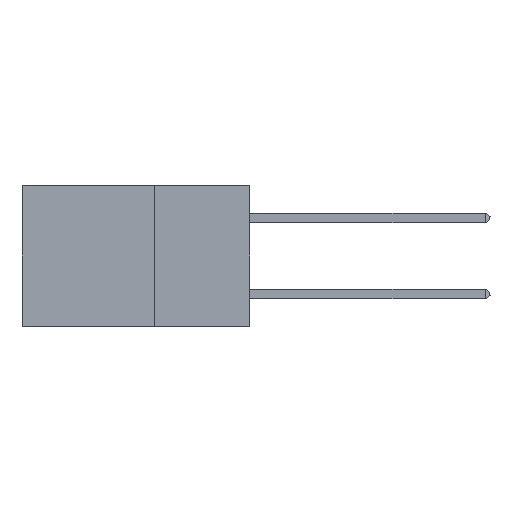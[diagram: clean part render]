
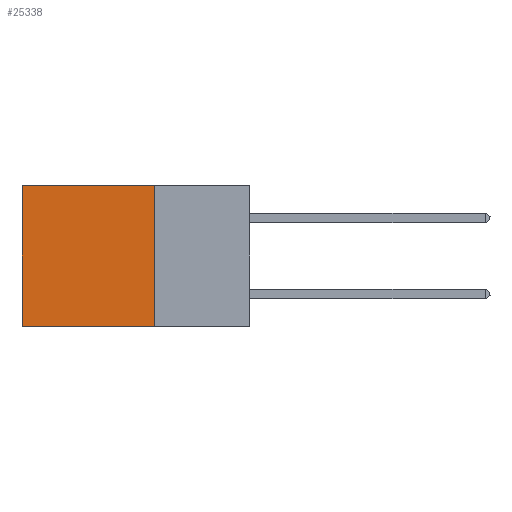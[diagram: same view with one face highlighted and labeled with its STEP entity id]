
A CAD part, left-side view. The second image highlights one B-rep face of the part: STEP entity #25338.
In plain terms, the highlighted planar face has unit normal (-1, 0, 0).
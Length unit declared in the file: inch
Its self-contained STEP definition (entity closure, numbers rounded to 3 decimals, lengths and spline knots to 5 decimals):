
#1166 = EDGE_CURVE ( 'NONE', #30699, #30476, #27440, .T. ) ;
#2408 = EDGE_CURVE ( 'NONE', #31710, #30699, #28452, .T. ) ;
#3236 = ORIENTED_EDGE ( 'NONE', *, *, #1166, .T. ) ;
#4123 = ORIENTED_EDGE ( 'NONE', *, *, #6733, .F. ) ;
#5353 = CARTESIAN_POINT ( 'NONE',  ( 0.2875, 0.25, 0. ) ) ;
#5544 = DIRECTION ( 'NONE',  ( 0., 0., -1. ) ) ;
#6733 = EDGE_CURVE ( 'NONE', #31710, #26208, #7927, .T. ) ;
#7927 = LINE ( 'NONE', #44238, #15707 ) ;
#9197 = VECTOR ( 'NONE', #19686, 39.37008 ) ;
#10017 = CARTESIAN_POINT ( 'NONE',  ( 0.2875, 0.6, 0. ) ) ;
#12684 = ORIENTED_EDGE ( 'NONE', *, *, #26432, .F. ) ;
#13459 = VECTOR ( 'NONE', #20202, 39.37008 ) ;
#15584 = AXIS2_PLACEMENT_3D ( 'NONE', #33986, #16617, #20193 ) ;
#15707 = VECTOR ( 'NONE', #5544, 39.37008 ) ;
#16617 = DIRECTION ( 'NONE',  ( 1., 0., 0. ) ) ;
#16790 = CARTESIAN_POINT ( 'NONE',  ( 0.2875, 0.25, -0.37 ) ) ;
#18431 = LINE ( 'NONE', #16790, #13459 ) ;
#18557 = FACE_OUTER_BOUND ( 'NONE', #42165, .T. ) ;
#19686 = DIRECTION ( 'NONE',  ( 0., 0., -1. ) ) ;
#19907 = CARTESIAN_POINT ( 'NONE',  ( 0.2875, 0.25, -0.37 ) ) ;
#20193 = DIRECTION ( 'NONE',  ( 0., 0., -1. ) ) ;
#20202 = DIRECTION ( 'NONE',  ( 0., 1., 0. ) ) ;
#20769 = ORIENTED_EDGE ( 'NONE', *, *, #2408, .T. ) ;
#25338 = ADVANCED_FACE ( 'NONE', ( #18557 ), #27615, .F. ) ;
#26208 = VERTEX_POINT ( 'NONE', #19907 ) ;
#26432 = EDGE_CURVE ( 'NONE', #26208, #30476, #18431, .T. ) ;
#27440 = LINE ( 'NONE', #40785, #9197 ) ;
#27615 = PLANE ( 'NONE',  #15584 ) ;
#28452 = LINE ( 'NONE', #40369, #34549 ) ;
#30476 = VERTEX_POINT ( 'NONE', #41348 ) ;
#30699 = VERTEX_POINT ( 'NONE', #10017 ) ;
#31710 = VERTEX_POINT ( 'NONE', #5353 ) ;
#33986 = CARTESIAN_POINT ( 'NONE',  ( 0.2875, 0.25, 0. ) ) ;
#34549 = VECTOR ( 'NONE', #43988, 39.37008 ) ;
#40369 = CARTESIAN_POINT ( 'NONE',  ( 0.2875, 0.25, 0. ) ) ;
#40785 = CARTESIAN_POINT ( 'NONE',  ( 0.2875, 0.6, 0. ) ) ;
#41348 = CARTESIAN_POINT ( 'NONE',  ( 0.2875, 0.6, -0.37 ) ) ;
#42165 = EDGE_LOOP ( 'NONE', ( #3236, #12684, #4123, #20769 ) ) ;
#43988 = DIRECTION ( 'NONE',  ( 0., 1., 0. ) ) ;
#44238 = CARTESIAN_POINT ( 'NONE',  ( 0.2875, 0.25, 0. ) ) ;
